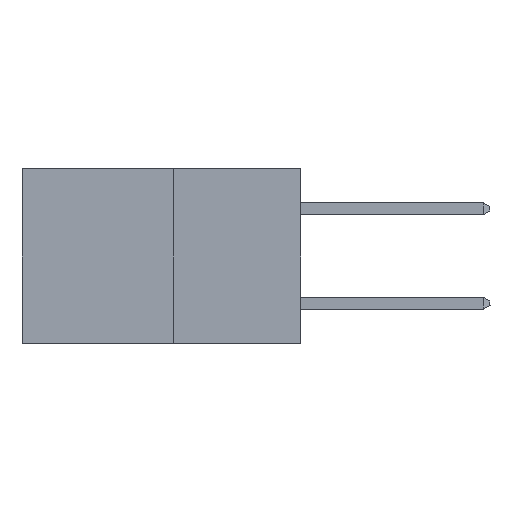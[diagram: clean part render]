
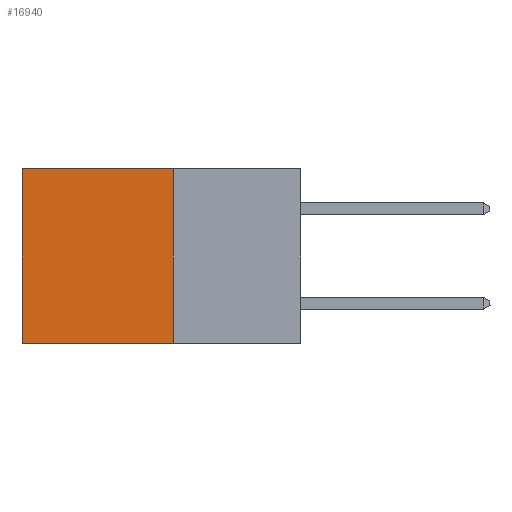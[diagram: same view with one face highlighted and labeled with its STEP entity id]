
A CAD part, left-side view. The second image highlights one B-rep face of the part: STEP entity #16940.
In plain terms, the highlighted planar face has unit normal (-1, 0, 0).
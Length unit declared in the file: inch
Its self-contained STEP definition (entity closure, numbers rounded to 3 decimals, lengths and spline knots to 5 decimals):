
#579 = CARTESIAN_POINT ( 'NONE',  ( 0.277, 0.27, 0. ) ) ;
#1202 = LINE ( 'NONE', #14376, #9563 ) ;
#1275 = EDGE_CURVE ( 'NONE', #12321, #19561, #14846, .T. ) ;
#2066 = VERTEX_POINT ( 'NONE', #579 ) ;
#2569 = LINE ( 'NONE', #17374, #6511 ) ;
#2836 = DIRECTION ( 'NONE',  ( 0., 0., -1. ) ) ;
#4159 = EDGE_LOOP ( 'NONE', ( #17099, #9391, #13766, #15833 ) ) ;
#6490 = EDGE_CURVE ( 'NONE', #2066, #11490, #6896, .T. ) ;
#6511 = VECTOR ( 'NONE', #17356, 39.37008 ) ;
#6896 = LINE ( 'NONE', #12881, #18979 ) ;
#7877 = AXIS2_PLACEMENT_3D ( 'NONE', #12741, #12807, #2836 ) ;
#8025 = CARTESIAN_POINT ( 'NONE',  ( 0.277, 0.59, 0. ) ) ;
#8971 = EDGE_CURVE ( 'NONE', #11490, #19561, #2569, .T. ) ;
#9391 = ORIENTED_EDGE ( 'NONE', *, *, #1275, .F. ) ;
#9563 = VECTOR ( 'NONE', #16034, 39.37008 ) ;
#10499 = VECTOR ( 'NONE', #14595, 39.37008 ) ;
#11400 = EDGE_CURVE ( 'NONE', #2066, #12321, #1202, .T. ) ;
#11490 = VERTEX_POINT ( 'NONE', #8025 ) ;
#11979 = CARTESIAN_POINT ( 'NONE',  ( 0.277, 0.27, -0.37 ) ) ;
#12321 = VERTEX_POINT ( 'NONE', #11979 ) ;
#12741 = CARTESIAN_POINT ( 'NONE',  ( 0.277, 0.27, -0.37 ) ) ;
#12807 = DIRECTION ( 'NONE',  ( 1., 0., 0. ) ) ;
#12809 = DIRECTION ( 'NONE',  ( 0., 1., 0. ) ) ;
#12881 = CARTESIAN_POINT ( 'NONE',  ( 0.277, 0.27, 0. ) ) ;
#13766 = ORIENTED_EDGE ( 'NONE', *, *, #11400, .F. ) ;
#14376 = CARTESIAN_POINT ( 'NONE',  ( 0.277, 0.27, -0.37 ) ) ;
#14595 = DIRECTION ( 'NONE',  ( 0., 1., 0. ) ) ;
#14846 = LINE ( 'NONE', #17463, #10499 ) ;
#15833 = ORIENTED_EDGE ( 'NONE', *, *, #6490, .T. ) ;
#16034 = DIRECTION ( 'NONE',  ( 0., 0., -1. ) ) ;
#16940 = ADVANCED_FACE ( 'NONE', ( #17222 ), #20892, .F. ) ;
#17099 = ORIENTED_EDGE ( 'NONE', *, *, #8971, .T. ) ;
#17222 = FACE_OUTER_BOUND ( 'NONE', #4159, .T. ) ;
#17356 = DIRECTION ( 'NONE',  ( 0., 0., -1. ) ) ;
#17374 = CARTESIAN_POINT ( 'NONE',  ( 0.277, 0.59, -0.37 ) ) ;
#17463 = CARTESIAN_POINT ( 'NONE',  ( 0.277, 0.27, -0.37 ) ) ;
#18979 = VECTOR ( 'NONE', #12809, 39.37008 ) ;
#19283 = CARTESIAN_POINT ( 'NONE',  ( 0.277, 0.59, -0.37 ) ) ;
#19561 = VERTEX_POINT ( 'NONE', #19283 ) ;
#20892 = PLANE ( 'NONE',  #7877 ) ;
